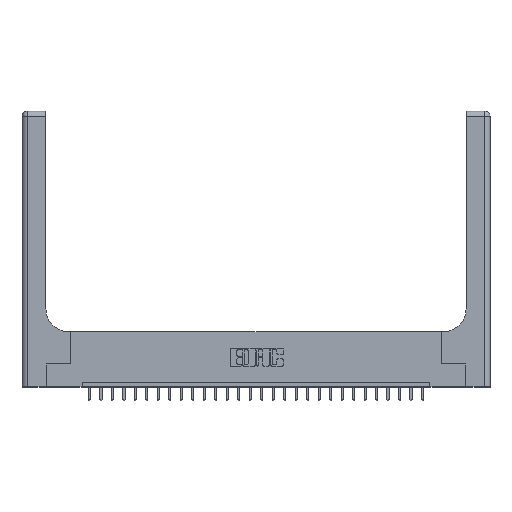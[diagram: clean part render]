
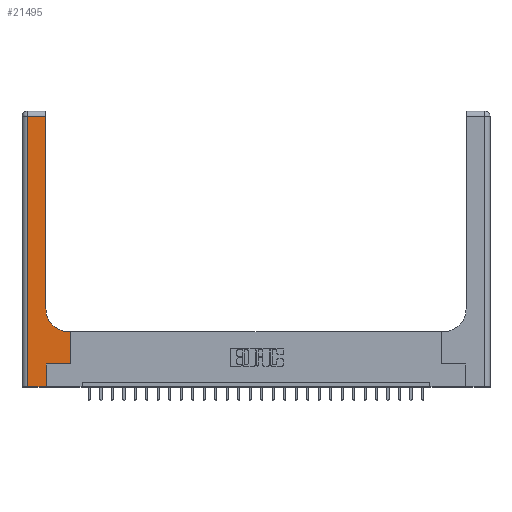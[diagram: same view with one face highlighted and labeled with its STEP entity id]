
A CAD part, top view. The second image highlights one B-rep face of the part: STEP entity #21495.
In plain terms, the highlighted planar face has unit normal (0, 0, 1).
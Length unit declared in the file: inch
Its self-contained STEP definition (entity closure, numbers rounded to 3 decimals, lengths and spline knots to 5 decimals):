
#435 = CARTESIAN_POINT ( 'NONE',  ( 0.265, 0.25, 0.37 ) ) ;
#656 = CARTESIAN_POINT ( 'NONE',  ( 0.528, 0.6, 0.37 ) ) ;
#674 = VERTEX_POINT ( 'NONE', #16632 ) ;
#1421 = EDGE_CURVE ( 'NONE', #22784, #7909, #7385, .T. ) ;
#1808 = VERTEX_POINT ( 'NONE', #13357 ) ;
#2461 = VERTEX_POINT ( 'NONE', #14863 ) ;
#2549 = DIRECTION ( 'NONE',  ( 0., 1., 0. ) ) ;
#2796 = CARTESIAN_POINT ( 'NONE',  ( 0.528, 0.25, 0.37 ) ) ;
#3061 = CARTESIAN_POINT ( 'NONE',  ( 0.528, 0.25, 0.37 ) ) ;
#3088 = EDGE_CURVE ( 'NONE', #1808, #674, #8039, .T. ) ;
#3189 = ORIENTED_EDGE ( 'NONE', *, *, #11030, .T. ) ;
#3737 = DIRECTION ( 'NONE',  ( 0., 0., -1. ) ) ;
#4026 = CARTESIAN_POINT ( 'NONE',  ( 0., 3., 0.37 ) ) ;
#4061 = DIRECTION ( 'NONE',  ( 0., 1., 0. ) ) ;
#4429 = VERTEX_POINT ( 'NONE', #3061 ) ;
#4463 = DIRECTION ( 'NONE',  ( 1., 0., 0. ) ) ;
#4493 = AXIS2_PLACEMENT_3D ( 'NONE', #21639, #3737, #19671 ) ;
#4803 = CARTESIAN_POINT ( 'NONE',  ( 0.51, 0.6, 0.37 ) ) ;
#4974 = EDGE_CURVE ( 'NONE', #10018, #2461, #15176, .T. ) ;
#5139 = EDGE_CURVE ( 'NONE', #4429, #20159, #20715, .T. ) ;
#5619 = DIRECTION ( 'NONE',  ( 0., -1., 0. ) ) ;
#5830 = DIRECTION ( 'NONE',  ( 0., 1., 0. ) ) ;
#6118 = PLANE ( 'NONE',  #6190 ) ;
#6190 = AXIS2_PLACEMENT_3D ( 'NONE', #4026, #25650, #15799 ) ;
#7085 = EDGE_CURVE ( 'NONE', #7909, #10018, #15695, .T. ) ;
#7248 = CARTESIAN_POINT ( 'NONE',  ( 0.26, 0.6, 0.37 ) ) ;
#7385 = CIRCLE ( 'NONE', #4493, 0.25 ) ;
#7506 = LINE ( 'NONE', #7248, #13766 ) ;
#7909 = VERTEX_POINT ( 'NONE', #13284 ) ;
#7929 = ORIENTED_EDGE ( 'NONE', *, *, #7085, .T. ) ;
#8039 = LINE ( 'NONE', #19798, #8404 ) ;
#8394 = LINE ( 'NONE', #435, #20090 ) ;
#8404 = VECTOR ( 'NONE', #5830, 39.37008 ) ;
#8851 = ORIENTED_EDGE ( 'NONE', *, *, #12970, .T. ) ;
#10018 = VERTEX_POINT ( 'NONE', #14454 ) ;
#11030 = EDGE_CURVE ( 'NONE', #13390, #1808, #12425, .T. ) ;
#11494 = LINE ( 'NONE', #19464, #20873 ) ;
#11759 = FACE_OUTER_BOUND ( 'NONE', #19797, .T. ) ;
#12167 = EDGE_CURVE ( 'NONE', #674, #4429, #8394, .T. ) ;
#12425 = LINE ( 'NONE', #20419, #25594 ) ;
#12477 = VECTOR ( 'NONE', #4061, 39.37008 ) ;
#12942 = CARTESIAN_POINT ( 'NONE',  ( 0., 2.94, 0.37 ) ) ;
#12970 = EDGE_CURVE ( 'NONE', #20159, #22784, #7506, .T. ) ;
#13284 = CARTESIAN_POINT ( 'NONE',  ( 0.26, 0.85, 0.37 ) ) ;
#13357 = CARTESIAN_POINT ( 'NONE',  ( 0.265, 0., 0.37 ) ) ;
#13377 = ORIENTED_EDGE ( 'NONE', *, *, #4974, .T. ) ;
#13390 = VERTEX_POINT ( 'NONE', #15810 ) ;
#13766 = VECTOR ( 'NONE', #21006, 39.37008 ) ;
#14454 = CARTESIAN_POINT ( 'NONE',  ( 0.26, 2.94, 0.37 ) ) ;
#14589 = ORIENTED_EDGE ( 'NONE', *, *, #3088, .T. ) ;
#14863 = CARTESIAN_POINT ( 'NONE',  ( 0.06, 2.94, 0.37 ) ) ;
#15176 = LINE ( 'NONE', #12942, #23071 ) ;
#15524 = ORIENTED_EDGE ( 'NONE', *, *, #12167, .T. ) ;
#15695 = LINE ( 'NONE', #23695, #12477 ) ;
#15799 = DIRECTION ( 'NONE',  ( -1., 0., 0. ) ) ;
#15810 = CARTESIAN_POINT ( 'NONE',  ( 0.06, 0., 0.37 ) ) ;
#16632 = CARTESIAN_POINT ( 'NONE',  ( 0.265, 0.25, 0.37 ) ) ;
#17313 = ORIENTED_EDGE ( 'NONE', *, *, #1421, .T. ) ;
#18697 = VECTOR ( 'NONE', #2549, 39.37008 ) ;
#19464 = CARTESIAN_POINT ( 'NONE',  ( 0.06, 3., 0.37 ) ) ;
#19671 = DIRECTION ( 'NONE',  ( 1., 0., 0. ) ) ;
#19791 = ORIENTED_EDGE ( 'NONE', *, *, #5139, .T. ) ;
#19797 = EDGE_LOOP ( 'NONE', ( #7929, #13377, #19895, #3189, #14589, #15524, #19791, #8851, #17313 ) ) ;
#19798 = CARTESIAN_POINT ( 'NONE',  ( 0.265, 0., 0.37 ) ) ;
#19895 = ORIENTED_EDGE ( 'NONE', *, *, #24212, .T. ) ;
#20090 = VECTOR ( 'NONE', #4463, 39.37008 ) ;
#20159 = VERTEX_POINT ( 'NONE', #656 ) ;
#20419 = CARTESIAN_POINT ( 'NONE',  ( 0., 0., 0.37 ) ) ;
#20715 = LINE ( 'NONE', #2796, #18697 ) ;
#20873 = VECTOR ( 'NONE', #5619, 39.37008 ) ;
#20947 = DIRECTION ( 'NONE',  ( -1., 0., 0. ) ) ;
#21006 = DIRECTION ( 'NONE',  ( -1., 0., 0. ) ) ;
#21495 = ADVANCED_FACE ( 'NONE', ( #11759 ), #6118, .F. ) ;
#21639 = CARTESIAN_POINT ( 'NONE',  ( 0.51, 0.85, 0.37 ) ) ;
#22784 = VERTEX_POINT ( 'NONE', #4803 ) ;
#23071 = VECTOR ( 'NONE', #20947, 39.37008 ) ;
#23695 = CARTESIAN_POINT ( 'NONE',  ( 0.26, 3., 0.37 ) ) ;
#24212 = EDGE_CURVE ( 'NONE', #2461, #13390, #11494, .T. ) ;
#24240 = DIRECTION ( 'NONE',  ( 1., 0., 0. ) ) ;
#25594 = VECTOR ( 'NONE', #24240, 39.37008 ) ;
#25650 = DIRECTION ( 'NONE',  ( 0., 0., -1. ) ) ;
